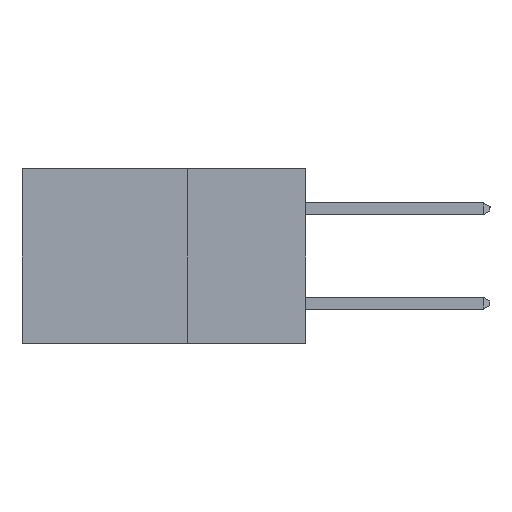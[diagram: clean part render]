
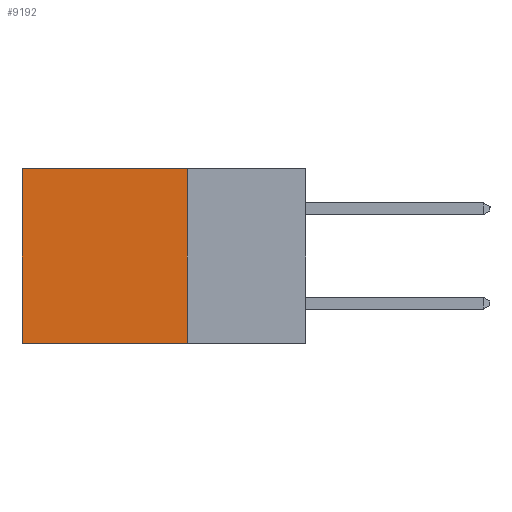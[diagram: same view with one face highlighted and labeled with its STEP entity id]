
A CAD part, left-side view. The second image highlights one B-rep face of the part: STEP entity #9192.
In plain terms, the highlighted planar face has unit normal (-1, 0, 0).
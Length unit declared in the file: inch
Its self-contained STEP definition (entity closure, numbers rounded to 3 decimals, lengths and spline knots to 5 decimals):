
#202 = CARTESIAN_POINT ( 'NONE',  ( 0.2615, 0.25, -0.37 ) ) ;
#907 = EDGE_CURVE ( 'NONE', #12589, #7602, #13032, .T. ) ;
#1108 = EDGE_CURVE ( 'NONE', #12589, #3941, #13538, .T. ) ;
#1166 = EDGE_CURVE ( 'NONE', #7602, #8304, #7039, .T. ) ;
#1378 = CARTESIAN_POINT ( 'NONE',  ( 0.2615, 0.25, -0.37 ) ) ;
#2732 = AXIS2_PLACEMENT_3D ( 'NONE', #202, #7217, #10665 ) ;
#3647 = CARTESIAN_POINT ( 'NONE',  ( 0.2615, 0.6, -0.37 ) ) ;
#3907 = VECTOR ( 'NONE', #12879, 39.37008 ) ;
#3941 = VERTEX_POINT ( 'NONE', #12791 ) ;
#4427 = EDGE_CURVE ( 'NONE', #3941, #8304, #13070, .T. ) ;
#5814 = EDGE_LOOP ( 'NONE', ( #12159, #9445, #9448, #10051 ) ) ;
#7039 = LINE ( 'NONE', #3647, #12670 ) ;
#7217 = DIRECTION ( 'NONE',  ( 1., 0., 0. ) ) ;
#7602 = VERTEX_POINT ( 'NONE', #8717 ) ;
#8304 = VERTEX_POINT ( 'NONE', #9440 ) ;
#8575 = VECTOR ( 'NONE', #9384, 39.37008 ) ;
#8717 = CARTESIAN_POINT ( 'NONE',  ( 0.2615, 0.6, 0. ) ) ;
#8813 = VECTOR ( 'NONE', #14674, 39.37008 ) ;
#9192 = ADVANCED_FACE ( 'NONE', ( #13835 ), #11498, .F. ) ;
#9336 = CARTESIAN_POINT ( 'NONE',  ( 0.2615, 0.25, 0. ) ) ;
#9384 = DIRECTION ( 'NONE',  ( 0., 1., 0. ) ) ;
#9440 = CARTESIAN_POINT ( 'NONE',  ( 0.2615, 0.6, -0.37 ) ) ;
#9445 = ORIENTED_EDGE ( 'NONE', *, *, #4427, .F. ) ;
#9448 = ORIENTED_EDGE ( 'NONE', *, *, #1108, .F. ) ;
#10051 = ORIENTED_EDGE ( 'NONE', *, *, #907, .T. ) ;
#10665 = DIRECTION ( 'NONE',  ( 0., 0., -1. ) ) ;
#11478 = DIRECTION ( 'NONE',  ( 0., 0., -1. ) ) ;
#11498 = PLANE ( 'NONE',  #2732 ) ;
#12159 = ORIENTED_EDGE ( 'NONE', *, *, #1166, .T. ) ;
#12589 = VERTEX_POINT ( 'NONE', #13375 ) ;
#12670 = VECTOR ( 'NONE', #11478, 39.37008 ) ;
#12791 = CARTESIAN_POINT ( 'NONE',  ( 0.2615, 0.25, -0.37 ) ) ;
#12879 = DIRECTION ( 'NONE',  ( 0., 1., 0. ) ) ;
#13007 = CARTESIAN_POINT ( 'NONE',  ( 0.2615, 0.25, -0.37 ) ) ;
#13032 = LINE ( 'NONE', #9336, #3907 ) ;
#13070 = LINE ( 'NONE', #13007, #8575 ) ;
#13375 = CARTESIAN_POINT ( 'NONE',  ( 0.2615, 0.25, 0. ) ) ;
#13538 = LINE ( 'NONE', #1378, #8813 ) ;
#13835 = FACE_OUTER_BOUND ( 'NONE', #5814, .T. ) ;
#14674 = DIRECTION ( 'NONE',  ( 0., 0., -1. ) ) ;
